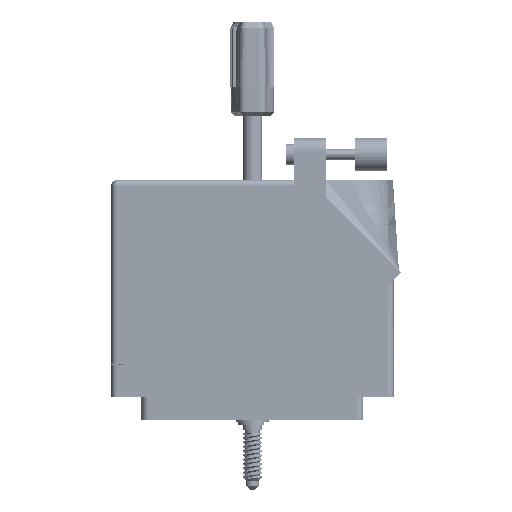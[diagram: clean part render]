
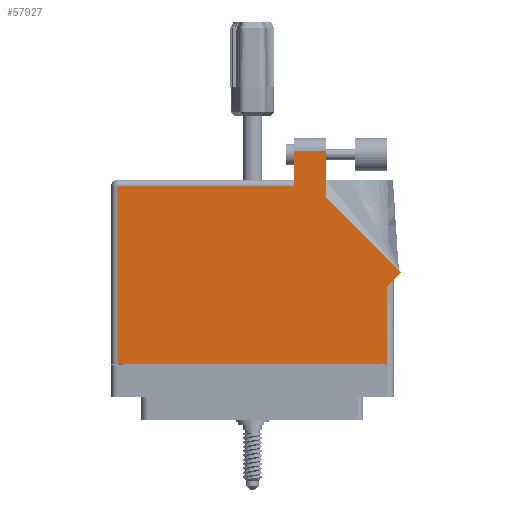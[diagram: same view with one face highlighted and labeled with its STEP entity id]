
A CAD part, front view. The second image highlights one B-rep face of the part: STEP entity #57927.
In plain terms, the highlighted face is planar.
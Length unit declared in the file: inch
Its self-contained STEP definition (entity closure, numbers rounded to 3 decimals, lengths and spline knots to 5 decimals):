
#1077 = CARTESIAN_POINT ( 'NONE',  ( 0.706, 1.95, 0.617 ) ) ;
#1577 = LINE ( 'NONE', #55203, #53153 ) ;
#2566 = EDGE_CURVE ( 'NONE', #20916, #69981, #41382, .T. ) ;
#3256 = VERTEX_POINT ( 'NONE', #71113 ) ;
#4225 = CARTESIAN_POINT ( 'NONE',  ( 0.399, 1.95, 0.617 ) ) ;
#6561 = VECTOR ( 'NONE', #81841, 39.37008 ) ;
#6741 = ORIENTED_EDGE ( 'NONE', *, *, #25720, .T. ) ;
#6852 = CARTESIAN_POINT ( 'NONE',  ( 1.42971, 0.78571, 0.617 ) ) ;
#7444 = VERTEX_POINT ( 'NONE', #41975 ) ;
#8590 = VERTEX_POINT ( 'NONE', #80253 ) ;
#9048 = CARTESIAN_POINT ( 'NONE',  ( 0.706, 1.50942, 0.617 ) ) ;
#11040 = LINE ( 'NONE', #37414, #85935 ) ;
#14597 = VECTOR ( 'NONE', #53022, 39.37008 ) ;
#15073 = VERTEX_POINT ( 'NONE', #65010 ) ;
#15252 = LINE ( 'NONE', #21833, #40108 ) ;
#20273 = VERTEX_POINT ( 'NONE', #23436 ) ;
#20916 = VERTEX_POINT ( 'NONE', #9048 ) ;
#21833 = CARTESIAN_POINT ( 'NONE',  ( 0.399, 1.675, 0.617 ) ) ;
#22060 = DIRECTION ( 'NONE',  ( 0., 1., 0. ) ) ;
#23436 = CARTESIAN_POINT ( 'NONE',  ( 1.297, 0.653, 0.617 ) ) ;
#24917 = LINE ( 'NONE', #4225, #14597 ) ;
#25720 = EDGE_CURVE ( 'NONE', #3256, #39457, #15252, .T. ) ;
#26937 = ORIENTED_EDGE ( 'NONE', *, *, #53921, .T. ) ;
#27816 = EDGE_LOOP ( 'NONE', ( #69243, #32671, #6741, #26937, #63016, #53312, #51414, #39663, #61421 ) ) ;
#32671 = ORIENTED_EDGE ( 'NONE', *, *, #83059, .T. ) ;
#32932 = CARTESIAN_POINT ( 'NONE',  ( -1.297, -0.1, 0.617 ) ) ;
#33488 = VECTOR ( 'NONE', #72347, 39.37008 ) ;
#34844 = CARTESIAN_POINT ( 'NONE',  ( -1.359, -0.1, 0.617 ) ) ;
#37414 = CARTESIAN_POINT ( 'NONE',  ( 1.359, 0.715, 0.617 ) ) ;
#38705 = EDGE_CURVE ( 'NONE', #7444, #43792, #43834, .T. ) ;
#39457 = VERTEX_POINT ( 'NONE', #60399 ) ;
#39663 = ORIENTED_EDGE ( 'NONE', *, *, #45712, .T. ) ;
#40108 = VECTOR ( 'NONE', #75428, 39.37008 ) ;
#40402 = EDGE_CURVE ( 'NONE', #8590, #20273, #1577, .T. ) ;
#41382 = LINE ( 'NONE', #68183, #59230 ) ;
#41975 = CARTESIAN_POINT ( 'NONE',  ( -1.297, 1.613, 0.617 ) ) ;
#43792 = VERTEX_POINT ( 'NONE', #32932 ) ;
#43834 = LINE ( 'NONE', #64916, #76949 ) ;
#45544 = LINE ( 'NONE', #6852, #33488 ) ;
#45712 = EDGE_CURVE ( 'NONE', #20273, #15073, #11040, .T. ) ;
#48340 = DIRECTION ( 'NONE',  ( -1., 0., 0. ) ) ;
#50003 = DIRECTION ( 'NONE',  ( 0., -1., 0. ) ) ;
#51256 = DIRECTION ( 'NONE',  ( -1., 0., 0. ) ) ;
#51414 = ORIENTED_EDGE ( 'NONE', *, *, #40402, .T. ) ;
#51903 = FACE_OUTER_BOUND ( 'NONE', #27816, .T. ) ;
#53022 = DIRECTION ( 'NONE',  ( -1., 0., 0. ) ) ;
#53153 = VECTOR ( 'NONE', #75413, 39.37008 ) ;
#53312 = ORIENTED_EDGE ( 'NONE', *, *, #54350, .T. ) ;
#53921 = EDGE_CURVE ( 'NONE', #39457, #7444, #57837, .T. ) ;
#54350 = EDGE_CURVE ( 'NONE', #43792, #8590, #67801, .T. ) ;
#55203 = CARTESIAN_POINT ( 'NONE',  ( 1.297, 0.715, 0.617 ) ) ;
#56315 = DIRECTION ( 'NONE',  ( 0.707, 0.707, 0. ) ) ;
#57837 = LINE ( 'NONE', #84641, #85086 ) ;
#57927 = ADVANCED_FACE ( 'NONE', ( #51903 ), #65522, .F. ) ;
#58925 = CARTESIAN_POINT ( 'NONE',  ( -1.359, 1.675, 0.617 ) ) ;
#59230 = VECTOR ( 'NONE', #22060, 39.37008 ) ;
#60399 = CARTESIAN_POINT ( 'NONE',  ( 0.399, 1.613, 0.617 ) ) ;
#61421 = ORIENTED_EDGE ( 'NONE', *, *, #66044, .T. ) ;
#61956 = DIRECTION ( 'NONE',  ( 0., 0., -1. ) ) ;
#63016 = ORIENTED_EDGE ( 'NONE', *, *, #38705, .T. ) ;
#64916 = CARTESIAN_POINT ( 'NONE',  ( -1.297, -0.1, 0.617 ) ) ;
#65010 = CARTESIAN_POINT ( 'NONE',  ( 1.42971, 0.78571, 0.617 ) ) ;
#65522 = PLANE ( 'NONE',  #85990 ) ;
#66044 = EDGE_CURVE ( 'NONE', #15073, #20916, #45544, .T. ) ;
#67801 = LINE ( 'NONE', #34844, #6561 ) ;
#68183 = CARTESIAN_POINT ( 'NONE',  ( 0.706, 1.50942, 0.617 ) ) ;
#69243 = ORIENTED_EDGE ( 'NONE', *, *, #2566, .T. ) ;
#69981 = VERTEX_POINT ( 'NONE', #1077 ) ;
#71113 = CARTESIAN_POINT ( 'NONE',  ( 0.399, 1.95, 0.617 ) ) ;
#72347 = DIRECTION ( 'NONE',  ( -0.707, 0.707, 0. ) ) ;
#75413 = DIRECTION ( 'NONE',  ( 0., 1., 0. ) ) ;
#75428 = DIRECTION ( 'NONE',  ( 0., -1., 0. ) ) ;
#76949 = VECTOR ( 'NONE', #50003, 39.37008 ) ;
#80253 = CARTESIAN_POINT ( 'NONE',  ( 1.297, -0.1, 0.617 ) ) ;
#81841 = DIRECTION ( 'NONE',  ( 1., 0., 0. ) ) ;
#83059 = EDGE_CURVE ( 'NONE', #69981, #3256, #24917, .T. ) ;
#84641 = CARTESIAN_POINT ( 'NONE',  ( -1.359, 1.613, 0.617 ) ) ;
#85086 = VECTOR ( 'NONE', #51256, 39.37008 ) ;
#85935 = VECTOR ( 'NONE', #56315, 39.37008 ) ;
#85990 = AXIS2_PLACEMENT_3D ( 'NONE', #58925, #61956, #48340 ) ;
